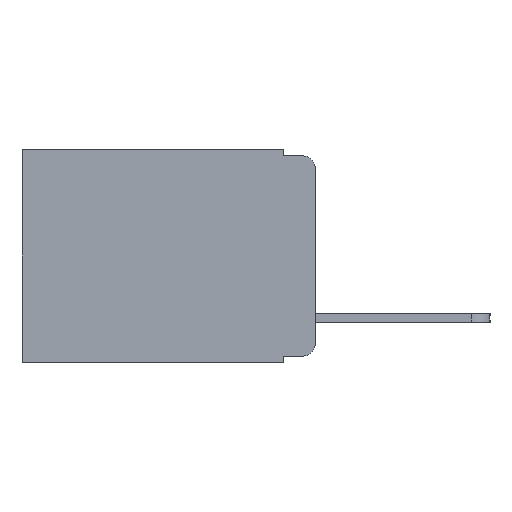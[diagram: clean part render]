
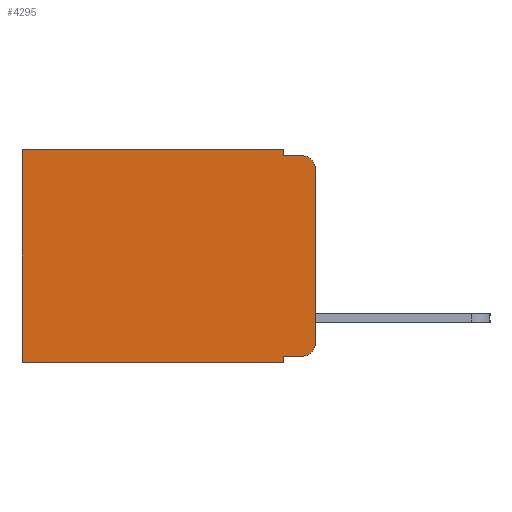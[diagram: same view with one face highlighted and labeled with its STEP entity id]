
A CAD part, left-side view. The second image highlights one B-rep face of the part: STEP entity #4295.
In plain terms, the highlighted planar face has unit normal (-1, 0, 0).
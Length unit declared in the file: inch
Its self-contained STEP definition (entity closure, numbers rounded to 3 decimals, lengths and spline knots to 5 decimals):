
#84 = LINE ( 'NONE', #19276, #12759 ) ;
#127 = EDGE_CURVE ( 'NONE', #18138, #271, #84, .T. ) ;
#156 = DIRECTION ( 'NONE',  ( 0., 0., -1. ) ) ;
#271 = VERTEX_POINT ( 'NONE', #5286 ) ;
#783 = ORIENTED_EDGE ( 'NONE', *, *, #3456, .T. ) ;
#803 = LINE ( 'NONE', #18009, #9272 ) ;
#1072 = VECTOR ( 'NONE', #11415, 39.37008 ) ;
#1184 = CARTESIAN_POINT ( 'NONE',  ( 0.298, 0.473, 0. ) ) ;
#1294 = ORIENTED_EDGE ( 'NONE', *, *, #2388, .F. ) ;
#1610 = DIRECTION ( 'NONE',  ( 1., 0., 0. ) ) ;
#1939 = VERTEX_POINT ( 'NONE', #16615 ) ;
#2329 = ORIENTED_EDGE ( 'NONE', *, *, #19223, .T. ) ;
#2388 = EDGE_CURVE ( 'NONE', #271, #1939, #15739, .T. ) ;
#2470 = CARTESIAN_POINT ( 'NONE',  ( 0.298, 0.473, -0.343 ) ) ;
#2602 = VECTOR ( 'NONE', #10493, 39.37008 ) ;
#2822 = ORIENTED_EDGE ( 'NONE', *, *, #17270, .T. ) ;
#2836 = CARTESIAN_POINT ( 'NONE',  ( 0.298, 0.051, 0. ) ) ;
#3190 = EDGE_LOOP ( 'NONE', ( #12868, #783, #1294, #13804, #14278, #2329, #6586, #18680, #2822, #19138 ) ) ;
#3383 = CARTESIAN_POINT ( 'NONE',  ( 0.298, 0., 0. ) ) ;
#3456 = EDGE_CURVE ( 'NONE', #11730, #1939, #3598, .T. ) ;
#3488 = VERTEX_POINT ( 'NONE', #5165 ) ;
#3598 = CIRCLE ( 'NONE', #16581, 0.02 ) ;
#3891 = CARTESIAN_POINT ( 'NONE',  ( 0.298, 0.02, -0.03 ) ) ;
#4274 = CARTESIAN_POINT ( 'NONE',  ( 0.298, 0.02, -0.333 ) ) ;
#4295 = ADVANCED_FACE ( 'NONE', ( #14016 ), #18025, .F. ) ;
#4381 = CARTESIAN_POINT ( 'NONE',  ( 0.298, 0.051, -0.01 ) ) ;
#5165 = CARTESIAN_POINT ( 'NONE',  ( 0.298, 0.051, -0.343 ) ) ;
#5286 = CARTESIAN_POINT ( 'NONE',  ( 0.298, 0.051, -0.01 ) ) ;
#5620 = CARTESIAN_POINT ( 'NONE',  ( 0.298, 0.02, -0.313 ) ) ;
#5632 = EDGE_CURVE ( 'NONE', #11730, #7309, #14666, .T. ) ;
#5725 = LINE ( 'NONE', #16086, #10092 ) ;
#6586 = ORIENTED_EDGE ( 'NONE', *, *, #17525, .F. ) ;
#6634 = CARTESIAN_POINT ( 'NONE',  ( 0.298, 0.051, 0. ) ) ;
#6903 = DIRECTION ( 'NONE',  ( 0., 0., -1. ) ) ;
#7197 = DIRECTION ( 'NONE',  ( 0., 0., -1. ) ) ;
#7309 = VERTEX_POINT ( 'NONE', #10904 ) ;
#7388 = CIRCLE ( 'NONE', #8889, 0.02 ) ;
#7592 = EDGE_CURVE ( 'NONE', #18138, #11841, #5725, .T. ) ;
#8601 = DIRECTION ( 'NONE',  ( 0., 0., -1. ) ) ;
#8889 = AXIS2_PLACEMENT_3D ( 'NONE', #5620, #16336, #7197 ) ;
#8908 = CARTESIAN_POINT ( 'NONE',  ( 0.298, 0.473, 0. ) ) ;
#8955 = DIRECTION ( 'NONE',  ( 0., 1., 0. ) ) ;
#8968 = CARTESIAN_POINT ( 'NONE',  ( 0.298, 0., 0. ) ) ;
#9198 = DIRECTION ( 'NONE',  ( 0., -1., 0. ) ) ;
#9272 = VECTOR ( 'NONE', #8955, 39.37008 ) ;
#9862 = CARTESIAN_POINT ( 'NONE',  ( 0.298, 0.051, -0.333 ) ) ;
#10035 = LINE ( 'NONE', #9862, #1072 ) ;
#10042 = VERTEX_POINT ( 'NONE', #12826 ) ;
#10092 = VECTOR ( 'NONE', #11628, 39.37008 ) ;
#10493 = DIRECTION ( 'NONE',  ( 0., 0., -1. ) ) ;
#10648 = VECTOR ( 'NONE', #12748, 39.37008 ) ;
#10711 = VECTOR ( 'NONE', #156, 39.37008 ) ;
#10904 = CARTESIAN_POINT ( 'NONE',  ( 0.298, 0., -0.313 ) ) ;
#11002 = LINE ( 'NONE', #8908, #2602 ) ;
#11056 = AXIS2_PLACEMENT_3D ( 'NONE', #8968, #1610, #12593 ) ;
#11415 = DIRECTION ( 'NONE',  ( 0., -1., 0. ) ) ;
#11628 = DIRECTION ( 'NONE',  ( 0., 1., 0. ) ) ;
#11730 = VERTEX_POINT ( 'NONE', #17909 ) ;
#11797 = VERTEX_POINT ( 'NONE', #4274 ) ;
#11841 = VERTEX_POINT ( 'NONE', #1184 ) ;
#12593 = DIRECTION ( 'NONE',  ( 0., 0., -1. ) ) ;
#12748 = DIRECTION ( 'NONE',  ( 0., 0., -1. ) ) ;
#12759 = VECTOR ( 'NONE', #6903, 39.37008 ) ;
#12826 = CARTESIAN_POINT ( 'NONE',  ( 0.298, 0.051, -0.333 ) ) ;
#12868 = ORIENTED_EDGE ( 'NONE', *, *, #5632, .F. ) ;
#13804 = ORIENTED_EDGE ( 'NONE', *, *, #127, .F. ) ;
#14016 = FACE_OUTER_BOUND ( 'NONE', #3190, .T. ) ;
#14278 = ORIENTED_EDGE ( 'NONE', *, *, #7592, .T. ) ;
#14666 = LINE ( 'NONE', #3383, #10648 ) ;
#14736 = DIRECTION ( 'NONE',  ( -1., 0., 0. ) ) ;
#15739 = LINE ( 'NONE', #4381, #17818 ) ;
#16086 = CARTESIAN_POINT ( 'NONE',  ( 0.298, 0., 0. ) ) ;
#16288 = EDGE_CURVE ( 'NONE', #11797, #7309, #7388, .T. ) ;
#16336 = DIRECTION ( 'NONE',  ( -1., 0., 0. ) ) ;
#16581 = AXIS2_PLACEMENT_3D ( 'NONE', #3891, #14736, #8601 ) ;
#16615 = CARTESIAN_POINT ( 'NONE',  ( 0.298, 0.02, -0.01 ) ) ;
#17270 = EDGE_CURVE ( 'NONE', #10042, #11797, #10035, .T. ) ;
#17525 = EDGE_CURVE ( 'NONE', #3488, #19175, #803, .T. ) ;
#17818 = VECTOR ( 'NONE', #9198, 39.37008 ) ;
#17909 = CARTESIAN_POINT ( 'NONE',  ( 0.298, 0., -0.03 ) ) ;
#18009 = CARTESIAN_POINT ( 'NONE',  ( 0.298, 0., -0.343 ) ) ;
#18025 = PLANE ( 'NONE',  #11056 ) ;
#18138 = VERTEX_POINT ( 'NONE', #2836 ) ;
#18237 = EDGE_CURVE ( 'NONE', #10042, #3488, #19118, .T. ) ;
#18680 = ORIENTED_EDGE ( 'NONE', *, *, #18237, .F. ) ;
#19118 = LINE ( 'NONE', #6634, #10711 ) ;
#19138 = ORIENTED_EDGE ( 'NONE', *, *, #16288, .T. ) ;
#19175 = VERTEX_POINT ( 'NONE', #2470 ) ;
#19223 = EDGE_CURVE ( 'NONE', #11841, #19175, #11002, .T. ) ;
#19276 = CARTESIAN_POINT ( 'NONE',  ( 0.298, 0.051, 0. ) ) ;
